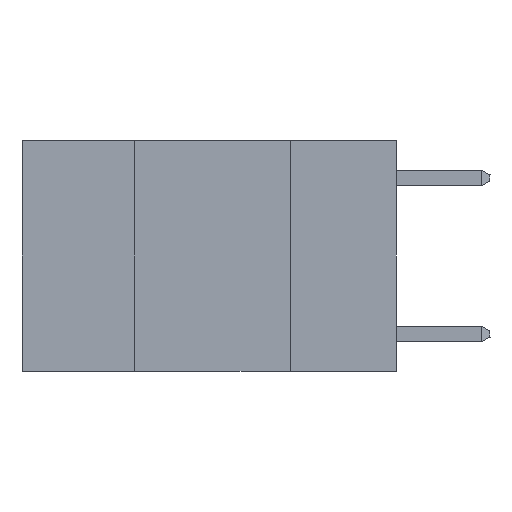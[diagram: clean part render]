
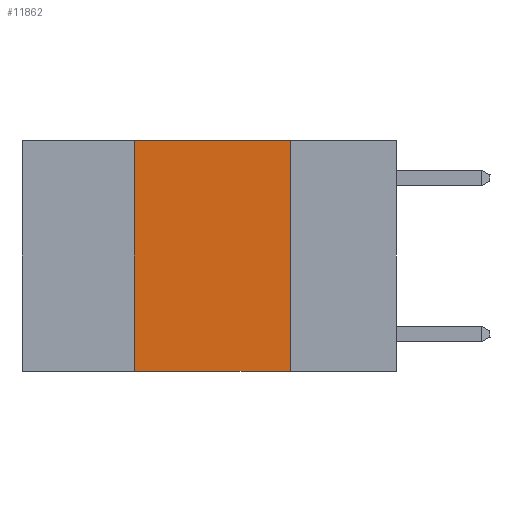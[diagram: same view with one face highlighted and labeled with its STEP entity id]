
A CAD part, left-side view. The second image highlights one B-rep face of the part: STEP entity #11862.
In plain terms, the highlighted planar face has unit normal (-1, 0, 0).
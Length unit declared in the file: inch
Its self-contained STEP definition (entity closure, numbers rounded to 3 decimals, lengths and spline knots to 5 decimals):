
#218 = VERTEX_POINT ( 'NONE', #10580 ) ;
#1139 = VECTOR ( 'NONE', #17091, 39.37008 ) ;
#1215 = EDGE_CURVE ( 'NONE', #12469, #218, #8266, .T. ) ;
#1821 = CARTESIAN_POINT ( 'NONE',  ( 0., 0.42, 0. ) ) ;
#3933 = DIRECTION ( 'NONE',  ( 0., 0., -1. ) ) ;
#4072 = VECTOR ( 'NONE', #9912, 39.37008 ) ;
#4133 = CARTESIAN_POINT ( 'NONE',  ( 0., 0.6, 0. ) ) ;
#5364 = DIRECTION ( 'NONE',  ( 0., -1., 0. ) ) ;
#6704 = LINE ( 'NONE', #16813, #1139 ) ;
#6748 = VECTOR ( 'NONE', #5364, 39.37008 ) ;
#6926 = VERTEX_POINT ( 'NONE', #12554 ) ;
#6979 = EDGE_LOOP ( 'NONE', ( #19072, #12232, #12730, #12740 ) ) ;
#7331 = CARTESIAN_POINT ( 'NONE',  ( 0., 0.42, -0.37 ) ) ;
#8073 = LINE ( 'NONE', #17005, #6748 ) ;
#8164 = EDGE_CURVE ( 'NONE', #6926, #218, #13148, .T. ) ;
#8266 = LINE ( 'NONE', #11490, #4072 ) ;
#9912 = DIRECTION ( 'NONE',  ( 0., -1., 0. ) ) ;
#10137 = PLANE ( 'NONE',  #13836 ) ;
#10249 = VERTEX_POINT ( 'NONE', #1821 ) ;
#10502 = DIRECTION ( 'NONE',  ( 0., 0., -1. ) ) ;
#10580 = CARTESIAN_POINT ( 'NONE',  ( 0., 0.17, -0.37 ) ) ;
#11490 = CARTESIAN_POINT ( 'NONE',  ( 0., 0.6, -0.37 ) ) ;
#11525 = DIRECTION ( 'NONE',  ( 1., 0., 0. ) ) ;
#11862 = ADVANCED_FACE ( 'NONE', ( #17427 ), #10137, .F. ) ;
#12232 = ORIENTED_EDGE ( 'NONE', *, *, #14555, .F. ) ;
#12292 = VECTOR ( 'NONE', #10502, 39.37008 ) ;
#12469 = VERTEX_POINT ( 'NONE', #7331 ) ;
#12554 = CARTESIAN_POINT ( 'NONE',  ( 0., 0.17, 0. ) ) ;
#12730 = ORIENTED_EDGE ( 'NONE', *, *, #13189, .F. ) ;
#12740 = ORIENTED_EDGE ( 'NONE', *, *, #1215, .T. ) ;
#13148 = LINE ( 'NONE', #14695, #12292 ) ;
#13189 = EDGE_CURVE ( 'NONE', #12469, #10249, #6704, .T. ) ;
#13836 = AXIS2_PLACEMENT_3D ( 'NONE', #4133, #11525, #3933 ) ;
#14555 = EDGE_CURVE ( 'NONE', #10249, #6926, #8073, .T. ) ;
#14695 = CARTESIAN_POINT ( 'NONE',  ( 0., 0.17, 0. ) ) ;
#16813 = CARTESIAN_POINT ( 'NONE',  ( 0., 0.42, 0. ) ) ;
#17005 = CARTESIAN_POINT ( 'NONE',  ( 0., 0.6, 0. ) ) ;
#17091 = DIRECTION ( 'NONE',  ( 0., 0., 1. ) ) ;
#17427 = FACE_OUTER_BOUND ( 'NONE', #6979, .T. ) ;
#19072 = ORIENTED_EDGE ( 'NONE', *, *, #8164, .F. ) ;
